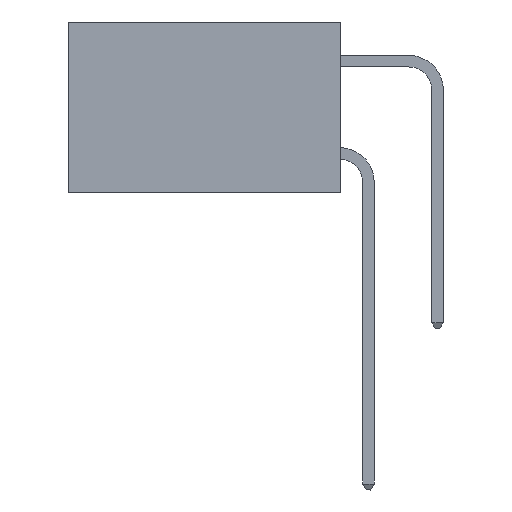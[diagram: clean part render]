
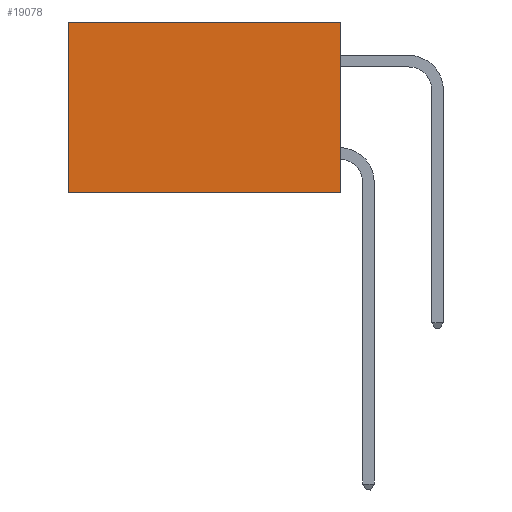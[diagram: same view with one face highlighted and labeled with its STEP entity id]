
A CAD part, left-side view. The second image highlights one B-rep face of the part: STEP entity #19078.
In plain terms, the highlighted planar face has unit normal (-1, 0, 0).
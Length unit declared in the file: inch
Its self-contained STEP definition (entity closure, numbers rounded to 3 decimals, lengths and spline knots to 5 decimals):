
#517 = CARTESIAN_POINT ( 'NONE',  ( 0.277, 0., -0.37 ) ) ;
#875 = VECTOR ( 'NONE', #12668, 39.37008 ) ;
#1078 = FACE_OUTER_BOUND ( 'NONE', #20604, .T. ) ;
#1859 = CARTESIAN_POINT ( 'NONE',  ( 0.277, 0.59, -0.37 ) ) ;
#2300 = CARTESIAN_POINT ( 'NONE',  ( 0.277, 0.59, -0.37 ) ) ;
#2482 = DIRECTION ( 'NONE',  ( 0., 0., -1. ) ) ;
#2919 = DIRECTION ( 'NONE',  ( 0., 0., -1. ) ) ;
#3087 = ORIENTED_EDGE ( 'NONE', *, *, #4819, .T. ) ;
#3935 = VERTEX_POINT ( 'NONE', #21050 ) ;
#4819 = EDGE_CURVE ( 'NONE', #3935, #29671, #20048, .T. ) ;
#6184 = VERTEX_POINT ( 'NONE', #2300 ) ;
#6805 = LINE ( 'NONE', #7633, #7561 ) ;
#7561 = VECTOR ( 'NONE', #2919, 39.37008 ) ;
#7633 = CARTESIAN_POINT ( 'NONE',  ( 0.277, 0., -0.37 ) ) ;
#9439 = EDGE_CURVE ( 'NONE', #3935, #21346, #6805, .T. ) ;
#9821 = CARTESIAN_POINT ( 'NONE',  ( 0.277, 0., 0. ) ) ;
#9824 = EDGE_CURVE ( 'NONE', #29671, #6184, #27373, .T. ) ;
#10650 = ORIENTED_EDGE ( 'NONE', *, *, #18182, .F. ) ;
#12177 = ORIENTED_EDGE ( 'NONE', *, *, #9439, .F. ) ;
#12375 = ORIENTED_EDGE ( 'NONE', *, *, #9824, .T. ) ;
#12469 = LINE ( 'NONE', #18693, #24418 ) ;
#12668 = DIRECTION ( 'NONE',  ( 0., 1., 0. ) ) ;
#14522 = PLANE ( 'NONE',  #23594 ) ;
#16304 = DIRECTION ( 'NONE',  ( 0., 1., 0. ) ) ;
#16890 = DIRECTION ( 'NONE',  ( 1., 0., 0. ) ) ;
#18182 = EDGE_CURVE ( 'NONE', #21346, #6184, #12469, .T. ) ;
#18693 = CARTESIAN_POINT ( 'NONE',  ( 0.277, 0., -0.37 ) ) ;
#19078 = ADVANCED_FACE ( 'NONE', ( #1078 ), #14522, .F. ) ;
#20048 = LINE ( 'NONE', #9821, #875 ) ;
#20604 = EDGE_LOOP ( 'NONE', ( #12375, #10650, #12177, #3087 ) ) ;
#21050 = CARTESIAN_POINT ( 'NONE',  ( 0.277, 0., 0. ) ) ;
#21346 = VERTEX_POINT ( 'NONE', #517 ) ;
#23594 = AXIS2_PLACEMENT_3D ( 'NONE', #23994, #16890, #2482 ) ;
#23994 = CARTESIAN_POINT ( 'NONE',  ( 0.277, 0., -0.37 ) ) ;
#24418 = VECTOR ( 'NONE', #16304, 39.37008 ) ;
#26624 = VECTOR ( 'NONE', #30527, 39.37008 ) ;
#27373 = LINE ( 'NONE', #1859, #26624 ) ;
#29671 = VERTEX_POINT ( 'NONE', #29677 ) ;
#29677 = CARTESIAN_POINT ( 'NONE',  ( 0.277, 0.59, 0. ) ) ;
#30527 = DIRECTION ( 'NONE',  ( 0., 0., -1. ) ) ;
